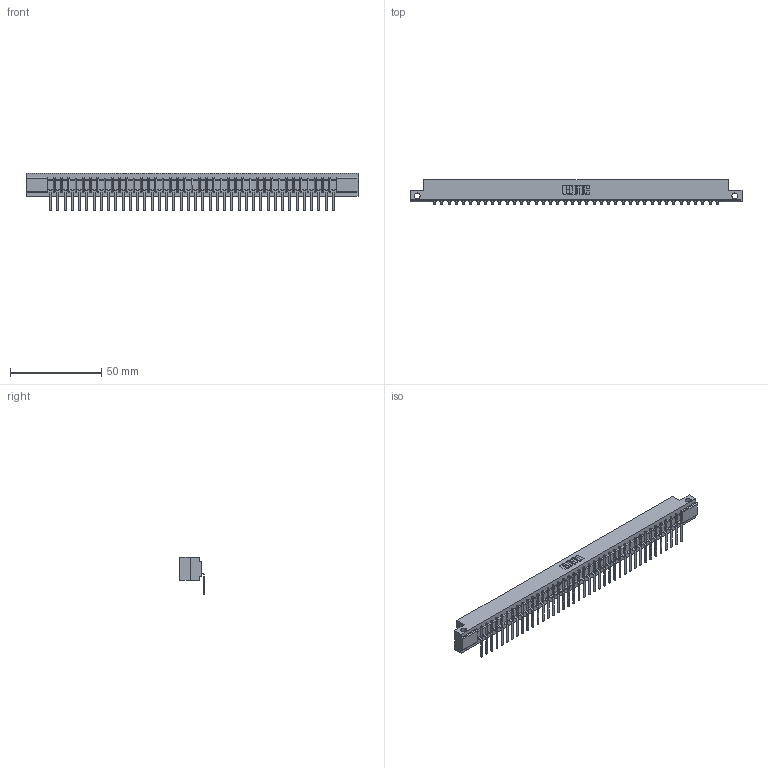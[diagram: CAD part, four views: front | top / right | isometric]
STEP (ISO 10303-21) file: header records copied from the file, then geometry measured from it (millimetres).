
FILE_DESCRIPTION (( 'STEP AP203' ), '1' );
FILE_NAME ('357-040-557-112.STEP', '2019-09-17T09:24:05', ( '' ), ( '' ), 'SwSTEP 2.0', 'SolidWorks 2016', '' );
FILE_SCHEMA (( 'CONFIG_CONTROL_DESIGN' ));
Length unit declared in the file: inch
Products named in the file (3): 307 Part_.128 Dia Side Mounting Holes; 307-290-002_557; 357-040-557-112
Assembly tree (41 placements, depth 2):
  357-040-557-112
    307 Part_.128 Dia Side Mounting Holes
    307-290-002_557  x40
Bounding box: 181.51 x 13.32 x 20.66 mm (x, y, z)
Volume: 19374.6 mm3; surface area: 25007.7 mm2
Topology: 41 solids, 41 shells, 3279 faces, 10083 edges, 6610 vertices
Faces by surface type: plane 1950, cylinder 1247, sphere 82
Entity records: 35394 total; most frequent: CARTESIAN_POINT 5972, ORIENTED_EDGE 5962, DIRECTION 5803, EDGE_CURVE 2981, LINE 2281, VECTOR 2281, VERTEX_POINT 1930, AXIS2_PLACEMENT_3D 1761
